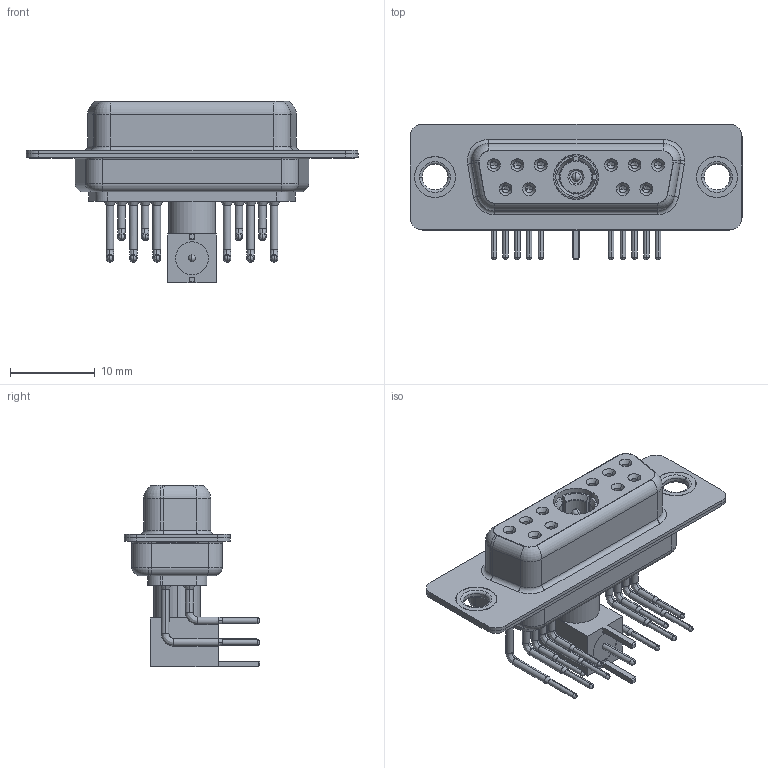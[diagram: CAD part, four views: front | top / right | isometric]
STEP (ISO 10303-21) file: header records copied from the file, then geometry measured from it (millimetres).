
FILE_DESCRIPTION (( 'STEP AP203' ), '1' );
FILE_NAME ('630-11W1240-7T1.STEP', '2022-05-31T10:11:35', ( '' ), ( '' ), 'SwSTEP 2.0', 'SolidWorks 2020', '' );
FILE_SCHEMA (( 'CONFIG_CONTROL_DESIGN' ));
Length unit declared in the file: millimetre
Products named in the file (14): 630-11W1240-7T1; Insulator RA Pin; Insulator Pin_Straight PC Tail; RA Back Shell; Pin_RA; 630Combo Shell Rear_15 Contacts; 630Combo Contact Row 2; Locking Collar; Co-Ax Plug_RA PC Tail; 630Combo Shell Front_15 Contacts; Co-Ax Plug Assy_RA; 630Combo Contact Row 1; 630Combo Thru Hole Rivet; 630Combo Housing_11W1
Assembly tree (22 placements, depth 3):
  630-11W1240-7T1
    630Combo Housing_11W1
    630Combo Shell Front_15 Contacts
    630Combo Shell Rear_15 Contacts
    630Combo Thru Hole Rivet  x2
    Co-Ax Plug Assy_RA
      Co-Ax Plug_RA PC Tail
      Insulator Pin_Straight PC Tail
      Pin_RA
      Locking Collar
      RA Back Shell
      Insulator RA Pin
    630Combo Contact Row 1  x6
    630Combo Contact Row 2  x4
Bounding box: 39.2 x 16 x 21.41 mm (x, y, z)
Volume: 2734.6 mm3; surface area: 6748.3 mm2
Topology: 21 solids, 21 shells, 951 faces, 2354 edges, 1472 vertices
Faces by surface type: cylinder 416, plane 284, cone 135, torus 71, bspline 41, sphere 4
Entity records: 19961 total; most frequent: CARTESIAN_POINT 3582, DIRECTION 3353, ORIENTED_EDGE 2876, EDGE_CURVE 1438, AXIS2_PLACEMENT_3D 1374, VERTEX_POINT 910, CIRCLE 746, EDGE_LOOP 714
